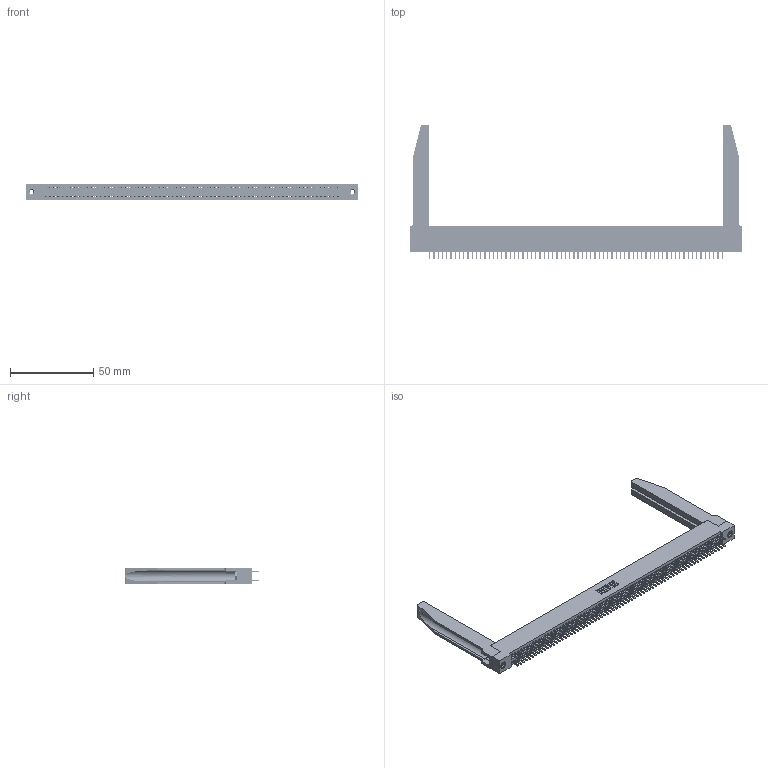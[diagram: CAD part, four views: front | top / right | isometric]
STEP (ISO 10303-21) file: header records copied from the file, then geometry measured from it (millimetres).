
FILE_DESCRIPTION (( 'STEP AP203' ), '1' );
FILE_NAME ('345-140-520-278.STEP', '2019-11-08T19:15:07', ( '' ), ( '' ), 'SwSTEP 2.0', 'SolidWorks 2016', '' );
FILE_SCHEMA (( 'CONFIG_CONTROL_DESIGN' ));
Length unit declared in the file: inch
Products named in the file (5): 345-292-001_345-293-120; 345-140-520-278; 345 Part_Flush Mounting Lugs - 0.156 Dia-TH; 345-250-001_345-250-001-102; 345-220-078_345-220-078
Assembly tree (145 placements, depth 2):
  345-140-520-278
    345 Part_Flush Mounting Lugs - 0.156 Dia-TH
    345-292-001_345-293-120  x140
    345-250-001_345-250-001-102  x2
    345-220-078_345-220-078  x2
Bounding box: 199.03 x 80.64 x 9.4 mm (x, y, z)
Volume: 27303.2 mm3; surface area: 36122.6 mm2
Topology: 145 solids, 145 shells, 7920 faces, 22929 edges, 14902 vertices
Faces by surface type: plane 5122, cylinder 2746, bspline 36, cone 12, torus 4
Entity records: 56008 total; most frequent: CARTESIAN_POINT 10291, ORIENTED_EDGE 9110, DIRECTION 8021, EDGE_CURVE 4555, LINE 4045, VECTOR 4045, VERTEX_POINT 3028, AXIS2_PLACEMENT_3D 1988
